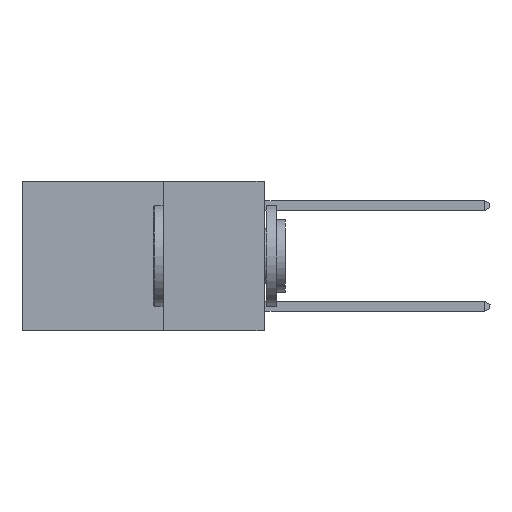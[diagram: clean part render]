
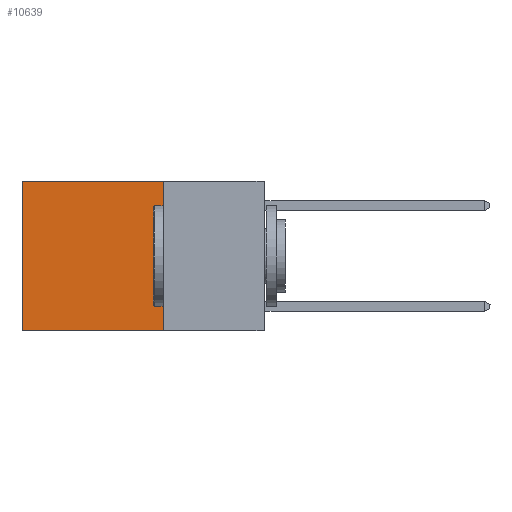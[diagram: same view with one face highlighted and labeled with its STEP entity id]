
A CAD part, left-side view. The second image highlights one B-rep face of the part: STEP entity #10639.
In plain terms, the highlighted planar face has unit normal (-1, 0, 0).
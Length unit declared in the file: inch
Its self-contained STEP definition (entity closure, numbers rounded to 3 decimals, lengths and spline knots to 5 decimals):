
#524 = VECTOR ( 'NONE', #5312, 39.37008 ) ;
#1592 = ORIENTED_EDGE ( 'NONE', *, *, #19857, .T. ) ;
#2398 = CARTESIAN_POINT ( 'NONE',  ( 0.2625, 0.6, -0.37 ) ) ;
#3482 = EDGE_LOOP ( 'NONE', ( #1592, #18035, #9174, #8430 ) ) ;
#3748 = EDGE_CURVE ( 'NONE', #12535, #9228, #19646, .T. ) ;
#4613 = LINE ( 'NONE', #15404, #524 ) ;
#5312 = DIRECTION ( 'NONE',  ( 0., 0., -1. ) ) ;
#5672 = DIRECTION ( 'NONE',  ( 0., 1., 0. ) ) ;
#5900 = CARTESIAN_POINT ( 'NONE',  ( 0.2625, 0.25, 0. ) ) ;
#6242 = VECTOR ( 'NONE', #11387, 39.37008 ) ;
#7170 = CARTESIAN_POINT ( 'NONE',  ( 0.2625, 0.25, 0. ) ) ;
#8052 = LINE ( 'NONE', #15759, #12523 ) ;
#8430 = ORIENTED_EDGE ( 'NONE', *, *, #3748, .T. ) ;
#8857 = DIRECTION ( 'NONE',  ( 0., 0., -1. ) ) ;
#9174 = ORIENTED_EDGE ( 'NONE', *, *, #15419, .F. ) ;
#9228 = VERTEX_POINT ( 'NONE', #9451 ) ;
#9451 = CARTESIAN_POINT ( 'NONE',  ( 0.2625, 0.6, 0. ) ) ;
#9502 = CARTESIAN_POINT ( 'NONE',  ( 0.2625, 0.25, 0. ) ) ;
#10639 = ADVANCED_FACE ( 'NONE', ( #18437 ), #19549, .F. ) ;
#11186 = DIRECTION ( 'NONE',  ( 0., 0., -1. ) ) ;
#11387 = DIRECTION ( 'NONE',  ( 0., 1., 0. ) ) ;
#12331 = CARTESIAN_POINT ( 'NONE',  ( 0.2625, 0.25, -0.37 ) ) ;
#12523 = VECTOR ( 'NONE', #5672, 39.37008 ) ;
#12535 = VERTEX_POINT ( 'NONE', #5900 ) ;
#13489 = EDGE_CURVE ( 'NONE', #16684, #16261, #8052, .T. ) ;
#14788 = AXIS2_PLACEMENT_3D ( 'NONE', #9502, #21211, #11186 ) ;
#15404 = CARTESIAN_POINT ( 'NONE',  ( 0.2625, 0.6, 0. ) ) ;
#15419 = EDGE_CURVE ( 'NONE', #12535, #16684, #16162, .T. ) ;
#15759 = CARTESIAN_POINT ( 'NONE',  ( 0.2625, 0.25, -0.37 ) ) ;
#16162 = LINE ( 'NONE', #7170, #20071 ) ;
#16261 = VERTEX_POINT ( 'NONE', #2398 ) ;
#16684 = VERTEX_POINT ( 'NONE', #12331 ) ;
#18035 = ORIENTED_EDGE ( 'NONE', *, *, #13489, .F. ) ;
#18069 = CARTESIAN_POINT ( 'NONE',  ( 0.2625, 0.25, 0. ) ) ;
#18437 = FACE_OUTER_BOUND ( 'NONE', #3482, .T. ) ;
#19549 = PLANE ( 'NONE',  #14788 ) ;
#19646 = LINE ( 'NONE', #18069, #6242 ) ;
#19857 = EDGE_CURVE ( 'NONE', #9228, #16261, #4613, .T. ) ;
#20071 = VECTOR ( 'NONE', #8857, 39.37008 ) ;
#21211 = DIRECTION ( 'NONE',  ( 1., 0., 0. ) ) ;
